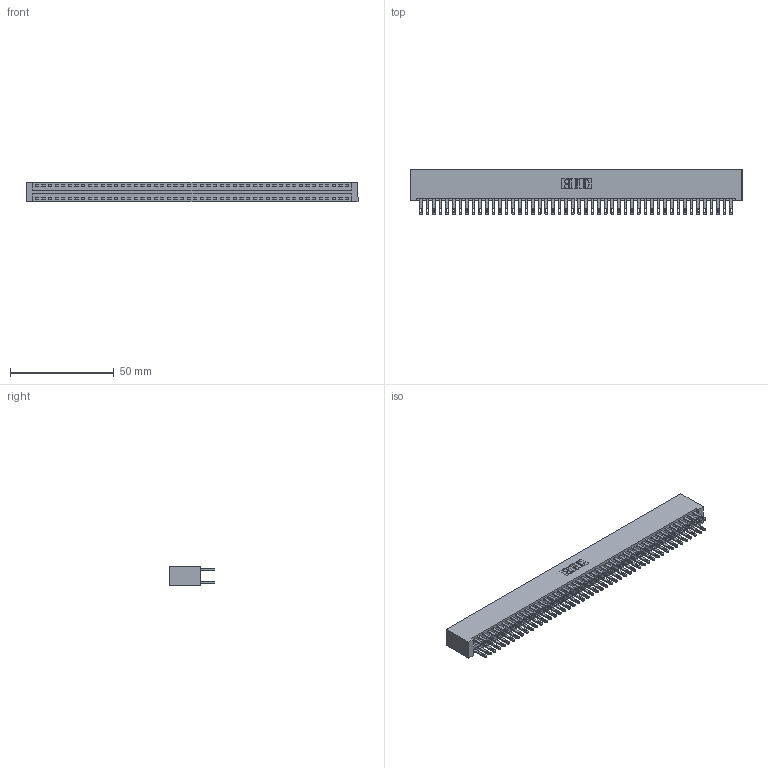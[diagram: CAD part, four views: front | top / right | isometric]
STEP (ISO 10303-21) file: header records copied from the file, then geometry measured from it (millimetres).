
FILE_DESCRIPTION (( 'STEP AP203' ), '1' );
FILE_NAME ('346-096-500-201.STEP', '2022-05-26T15:34:37', ( '' ), ( '' ), 'SwSTEP 2.0', 'SolidWorks 2020', '' );
FILE_SCHEMA (( 'CONFIG_CONTROL_DESIGN' ));
Length unit declared in the file: inch
Products named in the file (3): 345-292-001_345-293-100; 346-096-500-201; 346 Part_No Mounting Lugs
Assembly tree (97 placements, depth 2):
  346-096-500-201
    346 Part_No Mounting Lugs
    345-292-001_345-293-100  x96
Bounding box: 159.64 x 21.84 x 9.4 mm (x, y, z)
Volume: 16480 mm3; surface area: 23915.2 mm2
Topology: 97 solids, 97 shells, 4722 faces, 14417 edges, 9610 vertices
Faces by surface type: plane 2856, cylinder 1866
Entity records: 30171 total; most frequent: CARTESIAN_POINT 4960, ORIENTED_EDGE 4894, DIRECTION 4419, EDGE_CURVE 2447, VECTOR 2127, LINE 2127, VERTEX_POINT 1630, AXIS2_PLACEMENT_3D 1146
